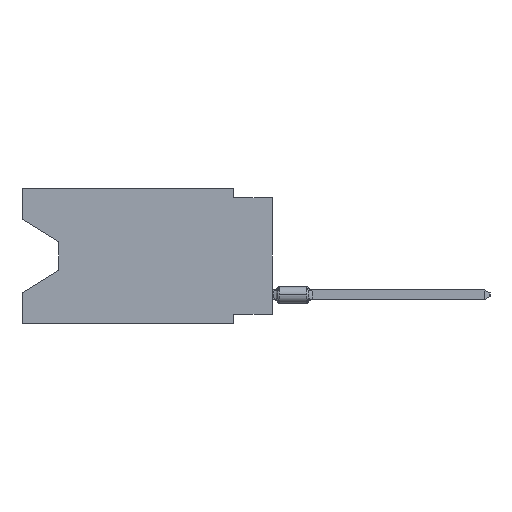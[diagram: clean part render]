
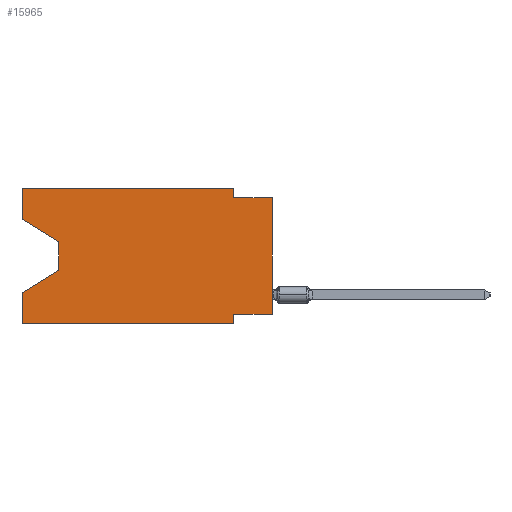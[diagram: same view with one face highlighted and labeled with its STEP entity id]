
A CAD part, left-side view. The second image highlights one B-rep face of the part: STEP entity #15965.
In plain terms, the highlighted planar face has unit normal (-1, 0, 0).
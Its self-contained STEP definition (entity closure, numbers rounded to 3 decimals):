
#270 = VERTEX_POINT ( 'NONE', #18604 ) ;
#402 = VERTEX_POINT ( 'NONE', #8827 ) ;
#418 = CARTESIAN_POINT ( 'NONE',  ( 0., 16.383, 0. ) ) ;
#1556 = CARTESIAN_POINT ( 'NONE',  ( 0., 13.97, -5.385 ) ) ;
#1591 = CARTESIAN_POINT ( 'NONE',  ( 0., 2.54, 0. ) ) ;
#1642 = VECTOR ( 'NONE', #17604, 1000. ) ;
#1862 = EDGE_CURVE ( 'NONE', #2423, #11524, #11014, .T. ) ;
#2329 = DIRECTION ( 'NONE',  ( 0., 0., 1. ) ) ;
#2419 = CARTESIAN_POINT ( 'NONE',  ( 0., 2.54, 0. ) ) ;
#2423 = VERTEX_POINT ( 'NONE', #10003 ) ;
#3504 = EDGE_CURVE ( 'NONE', #7897, #9102, #4269, .T. ) ;
#3580 = CARTESIAN_POINT ( 'NONE',  ( 0., 16.383, -6.852 ) ) ;
#3996 = CARTESIAN_POINT ( 'NONE',  ( 0., 0., -0.635 ) ) ;
#4256 = LINE ( 'NONE', #1591, #26097 ) ;
#4269 = LINE ( 'NONE', #6590, #1642 ) ;
#4692 = ORIENTED_EDGE ( 'NONE', *, *, #22679, .F. ) ;
#5040 = DIRECTION ( 'NONE',  ( 0., 0., 1. ) ) ;
#5405 = LINE ( 'NONE', #27621, #34503 ) ;
#5421 = ORIENTED_EDGE ( 'NONE', *, *, #11927, .F. ) ;
#5699 = CARTESIAN_POINT ( 'NONE',  ( 0., 16.383, 0. ) ) ;
#5764 = DIRECTION ( 'NONE',  ( 0., -1., 0. ) ) ;
#5842 = VERTEX_POINT ( 'NONE', #12440 ) ;
#6197 = CARTESIAN_POINT ( 'NONE',  ( 0., 16.383, 0. ) ) ;
#6536 = VECTOR ( 'NONE', #31201, 1000. ) ;
#6590 = CARTESIAN_POINT ( 'NONE',  ( 0., 13.97, -5.385 ) ) ;
#6835 = LINE ( 'NONE', #3996, #6536 ) ;
#7897 = VERTEX_POINT ( 'NONE', #1556 ) ;
#7930 = LINE ( 'NONE', #13431, #34958 ) ;
#8279 = VECTOR ( 'NONE', #33063, 1000. ) ;
#8370 = DIRECTION ( 'NONE',  ( 0., -1., 0. ) ) ;
#8599 = CARTESIAN_POINT ( 'NONE',  ( 0., 2.54, -8.89 ) ) ;
#8694 = ORIENTED_EDGE ( 'NONE', *, *, #16796, .T. ) ;
#8827 = CARTESIAN_POINT ( 'NONE',  ( 0., 16.383, -8.89 ) ) ;
#9086 = VECTOR ( 'NONE', #16340, 1000. ) ;
#9102 = VERTEX_POINT ( 'NONE', #3580 ) ;
#9574 = EDGE_CURVE ( 'NONE', #2423, #10573, #10201, .T. ) ;
#9712 = VERTEX_POINT ( 'NONE', #8599 ) ;
#9922 = DIRECTION ( 'NONE',  ( 0., 1., 0. ) ) ;
#10003 = CARTESIAN_POINT ( 'NONE',  ( 0., 16.383, -2.038 ) ) ;
#10201 = LINE ( 'NONE', #18894, #14998 ) ;
#10573 = VERTEX_POINT ( 'NONE', #19872 ) ;
#10896 = ORIENTED_EDGE ( 'NONE', *, *, #15055, .F. ) ;
#11014 = LINE ( 'NONE', #6197, #9086 ) ;
#11220 = EDGE_CURVE ( 'NONE', #270, #28708, #6835, .T. ) ;
#11368 = CARTESIAN_POINT ( 'NONE',  ( 0., 13.97, -3.505 ) ) ;
#11524 = VERTEX_POINT ( 'NONE', #418 ) ;
#11927 = EDGE_CURVE ( 'NONE', #402, #9102, #27223, .T. ) ;
#12440 = CARTESIAN_POINT ( 'NONE',  ( 0., 2.54, -8.255 ) ) ;
#12747 = EDGE_CURVE ( 'NONE', #11524, #14428, #30753, .T. ) ;
#12760 = LINE ( 'NONE', #17914, #24292 ) ;
#13172 = EDGE_CURVE ( 'NONE', #5842, #9712, #7930, .T. ) ;
#13431 = CARTESIAN_POINT ( 'NONE',  ( 0., 2.54, -8.89 ) ) ;
#13597 = EDGE_CURVE ( 'NONE', #29335, #28708, #23722, .T. ) ;
#14032 = ORIENTED_EDGE ( 'NONE', *, *, #12747, .F. ) ;
#14428 = VERTEX_POINT ( 'NONE', #2419 ) ;
#14508 = ORIENTED_EDGE ( 'NONE', *, *, #31391, .T. ) ;
#14998 = VECTOR ( 'NONE', #21225, 1000. ) ;
#15055 = EDGE_CURVE ( 'NONE', #29335, #5842, #12760, .T. ) ;
#15965 = ADVANCED_FACE ( 'NONE', ( #21526 ), #32904, .F. ) ;
#16340 = DIRECTION ( 'NONE',  ( 0., 0., 1. ) ) ;
#16616 = EDGE_LOOP ( 'NONE', ( #19525, #8694, #17471, #5421, #14508, #30619, #10896, #31070, #17017, #4692, #14032, #21554 ) ) ;
#16796 = EDGE_CURVE ( 'NONE', #10573, #7897, #25772, .T. ) ;
#17017 = ORIENTED_EDGE ( 'NONE', *, *, #11220, .F. ) ;
#17471 = ORIENTED_EDGE ( 'NONE', *, *, #3504, .T. ) ;
#17604 = DIRECTION ( 'NONE',  ( 0., 0.855, -0.519 ) ) ;
#17914 = CARTESIAN_POINT ( 'NONE',  ( 0., 0., -8.255 ) ) ;
#18604 = CARTESIAN_POINT ( 'NONE',  ( 0., 2.54, -0.635 ) ) ;
#18894 = CARTESIAN_POINT ( 'NONE',  ( 0., 16.383, -2.038 ) ) ;
#19525 = ORIENTED_EDGE ( 'NONE', *, *, #9574, .T. ) ;
#19872 = CARTESIAN_POINT ( 'NONE',  ( 0., 13.97, -3.505 ) ) ;
#19907 = CARTESIAN_POINT ( 'NONE',  ( 0., 16.383, 0. ) ) ;
#21225 = DIRECTION ( 'NONE',  ( 0., -0.855, -0.519 ) ) ;
#21526 = FACE_OUTER_BOUND ( 'NONE', #16616, .T. ) ;
#21554 = ORIENTED_EDGE ( 'NONE', *, *, #1862, .F. ) ;
#22679 = EDGE_CURVE ( 'NONE', #14428, #270, #4256, .T. ) ;
#23462 = DIRECTION ( 'NONE',  ( 0., 0., -1. ) ) ;
#23722 = LINE ( 'NONE', #26564, #25335 ) ;
#24026 = CARTESIAN_POINT ( 'NONE',  ( 0., 16.383, 0. ) ) ;
#24292 = VECTOR ( 'NONE', #9922, 1000. ) ;
#25335 = VECTOR ( 'NONE', #5040, 1000. ) ;
#25772 = LINE ( 'NONE', #11368, #8279 ) ;
#26097 = VECTOR ( 'NONE', #23462, 1000. ) ;
#26564 = CARTESIAN_POINT ( 'NONE',  ( 0., 0., 0. ) ) ;
#27223 = LINE ( 'NONE', #24026, #32071 ) ;
#27621 = CARTESIAN_POINT ( 'NONE',  ( 0., 16.383, -8.89 ) ) ;
#27733 = AXIS2_PLACEMENT_3D ( 'NONE', #5699, #35027, #30048 ) ;
#28140 = VECTOR ( 'NONE', #8370, 1000. ) ;
#28708 = VERTEX_POINT ( 'NONE', #31673 ) ;
#29335 = VERTEX_POINT ( 'NONE', #30361 ) ;
#30048 = DIRECTION ( 'NONE',  ( 0., 0., -1. ) ) ;
#30361 = CARTESIAN_POINT ( 'NONE',  ( 0., 0., -8.255 ) ) ;
#30619 = ORIENTED_EDGE ( 'NONE', *, *, #13172, .F. ) ;
#30753 = LINE ( 'NONE', #19907, #28140 ) ;
#31070 = ORIENTED_EDGE ( 'NONE', *, *, #13597, .T. ) ;
#31201 = DIRECTION ( 'NONE',  ( 0., -1., 0. ) ) ;
#31391 = EDGE_CURVE ( 'NONE', #402, #9712, #5405, .T. ) ;
#31673 = CARTESIAN_POINT ( 'NONE',  ( 0., 0., -0.635 ) ) ;
#32071 = VECTOR ( 'NONE', #2329, 1000. ) ;
#32904 = PLANE ( 'NONE',  #27733 ) ;
#33063 = DIRECTION ( 'NONE',  ( 0., 0., -1. ) ) ;
#34503 = VECTOR ( 'NONE', #5764, 1000. ) ;
#34603 = DIRECTION ( 'NONE',  ( 0., 0., -1. ) ) ;
#34958 = VECTOR ( 'NONE', #34603, 1000. ) ;
#35027 = DIRECTION ( 'NONE',  ( 1., 0., 0. ) ) ;
